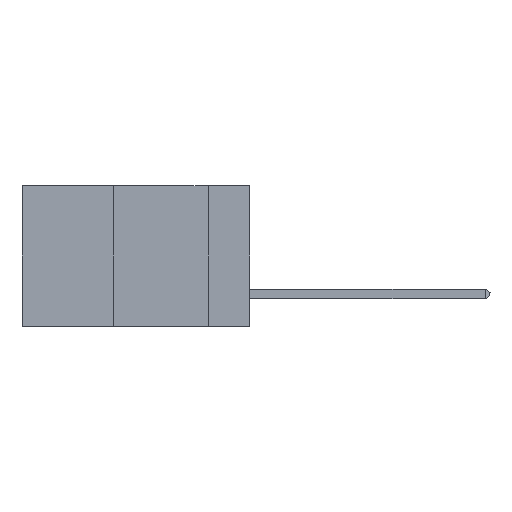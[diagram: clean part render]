
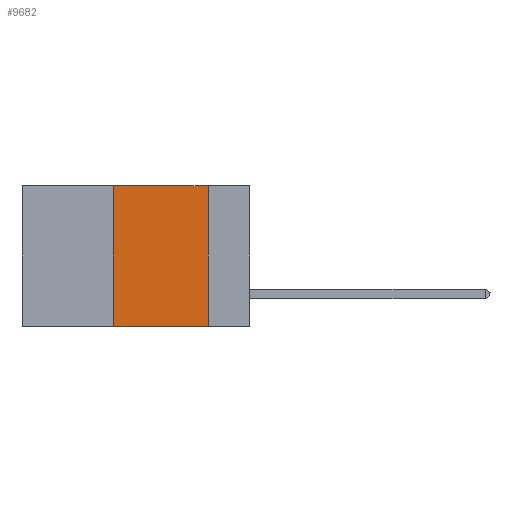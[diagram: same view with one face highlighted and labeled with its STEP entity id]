
A CAD part, left-side view. The second image highlights one B-rep face of the part: STEP entity #9682.
In plain terms, the highlighted planar face has unit normal (-1, 0, 0).
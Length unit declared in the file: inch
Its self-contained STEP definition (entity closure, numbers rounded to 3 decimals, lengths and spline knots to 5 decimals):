
#12 = EDGE_LOOP ( 'NONE', ( #26059, #6541, #1089, #3048 ) ) ;
#566 = VECTOR ( 'NONE', #6785, 39.37008 ) ;
#875 = VERTEX_POINT ( 'NONE', #32948 ) ;
#1089 = ORIENTED_EDGE ( 'NONE', *, *, #19975, .F. ) ;
#2220 = AXIS2_PLACEMENT_3D ( 'NONE', #3906, #14593, #14730 ) ;
#3048 = ORIENTED_EDGE ( 'NONE', *, *, #31773, .T. ) ;
#3906 = CARTESIAN_POINT ( 'NONE',  ( 0., 0.6, 0. ) ) ;
#4623 = FACE_OUTER_BOUND ( 'NONE', #12, .T. ) ;
#6541 = ORIENTED_EDGE ( 'NONE', *, *, #12674, .F. ) ;
#6785 = DIRECTION ( 'NONE',  ( 0., -1., 0. ) ) ;
#7369 = CARTESIAN_POINT ( 'NONE',  ( 0., 0.11, -0.37 ) ) ;
#8616 = CARTESIAN_POINT ( 'NONE',  ( 0., 0.36, 0. ) ) ;
#8909 = CARTESIAN_POINT ( 'NONE',  ( 0., 0.6, 0. ) ) ;
#9682 = ADVANCED_FACE ( 'NONE', ( #4623 ), #11908, .F. ) ;
#9915 = LINE ( 'NONE', #8909, #22505 ) ;
#10379 = VECTOR ( 'NONE', #27675, 39.37008 ) ;
#10705 = LINE ( 'NONE', #13530, #566 ) ;
#11908 = PLANE ( 'NONE',  #2220 ) ;
#12674 = EDGE_CURVE ( 'NONE', #32456, #15356, #9915, .T. ) ;
#13530 = CARTESIAN_POINT ( 'NONE',  ( 0., 0.6, -0.37 ) ) ;
#14054 = VERTEX_POINT ( 'NONE', #7369 ) ;
#14593 = DIRECTION ( 'NONE',  ( 1., 0., 0. ) ) ;
#14730 = DIRECTION ( 'NONE',  ( 0., 0., -1. ) ) ;
#15356 = VERTEX_POINT ( 'NONE', #26584 ) ;
#17291 = LINE ( 'NONE', #23217, #26499 ) ;
#19975 = EDGE_CURVE ( 'NONE', #875, #32456, #17291, .T. ) ;
#21143 = DIRECTION ( 'NONE',  ( 0., -1., 0. ) ) ;
#22367 = EDGE_CURVE ( 'NONE', #15356, #14054, #33008, .T. ) ;
#22505 = VECTOR ( 'NONE', #21143, 39.37008 ) ;
#23217 = CARTESIAN_POINT ( 'NONE',  ( 0., 0.36, 0. ) ) ;
#26059 = ORIENTED_EDGE ( 'NONE', *, *, #22367, .F. ) ;
#26499 = VECTOR ( 'NONE', #30292, 39.37008 ) ;
#26584 = CARTESIAN_POINT ( 'NONE',  ( 0., 0.11, 0. ) ) ;
#27675 = DIRECTION ( 'NONE',  ( 0., 0., -1. ) ) ;
#30243 = CARTESIAN_POINT ( 'NONE',  ( 0., 0.11, 0. ) ) ;
#30292 = DIRECTION ( 'NONE',  ( 0., 0., 1. ) ) ;
#31773 = EDGE_CURVE ( 'NONE', #875, #14054, #10705, .T. ) ;
#32456 = VERTEX_POINT ( 'NONE', #8616 ) ;
#32948 = CARTESIAN_POINT ( 'NONE',  ( 0., 0.36, -0.37 ) ) ;
#33008 = LINE ( 'NONE', #30243, #10379 ) ;
